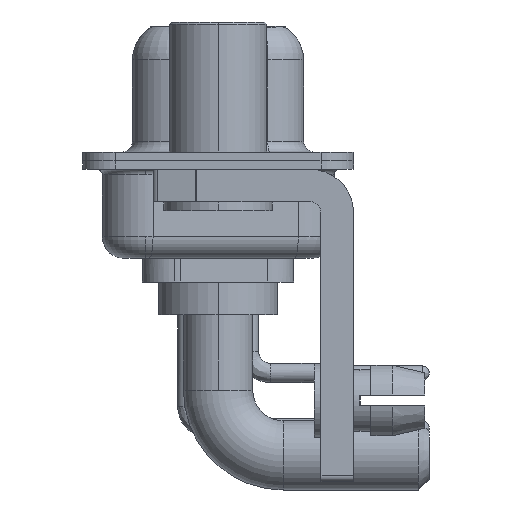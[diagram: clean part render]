
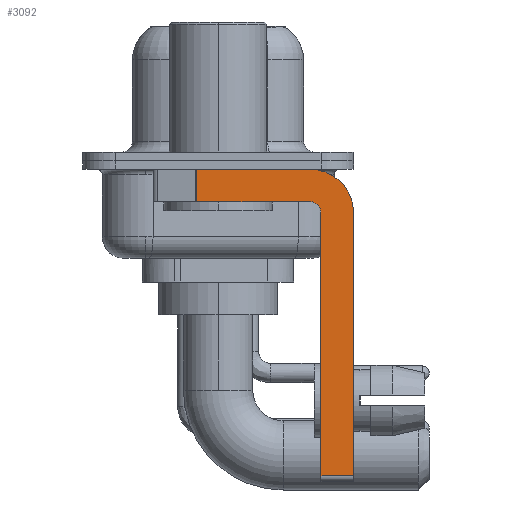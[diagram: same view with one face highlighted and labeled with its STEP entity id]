
A CAD part, left-side view. The second image highlights one B-rep face of the part: STEP entity #3092.
In plain terms, the highlighted planar face has unit normal (-1, 0, 0).
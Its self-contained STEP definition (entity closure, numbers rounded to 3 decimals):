
#45 = ORIENTED_EDGE ( 'NONE', *, *, #5757, .F. ) ;
#236 = LINE ( 'NONE', #1797, #17613 ) ;
#726 = CARTESIAN_POINT ( 'NONE',  ( -2.9, -4.25, -0.4 ) ) ;
#1777 = VERTEX_POINT ( 'NONE', #4942 ) ;
#1797 = CARTESIAN_POINT ( 'NONE',  ( -2.9, -4.25, -1.9 ) ) ;
#2208 = DIRECTION ( 'NONE',  ( 0., 0., -1. ) ) ;
#2331 = CIRCLE ( 'NONE', #6593, 2. ) ;
#2436 = EDGE_LOOP ( 'NONE', ( #10477, #22386, #17384, #18228, #45, #11481, #5623, #11283 ) ) ;
#3092 = ADVANCED_FACE ( 'NONE', ( #6260 ), #6143, .F. ) ;
#3889 = CARTESIAN_POINT ( 'NONE',  ( -2.9, -4.25, -14.55 ) ) ;
#4396 = VECTOR ( 'NONE', #17489, 1000. ) ;
#4942 = CARTESIAN_POINT ( 'NONE',  ( -2.9, -4.25, -1.9 ) ) ;
#5421 = DIRECTION ( 'NONE',  ( 0., 1., 0. ) ) ;
#5623 = ORIENTED_EDGE ( 'NONE', *, *, #12557, .F. ) ;
#5757 = EDGE_CURVE ( 'NONE', #8678, #9467, #18134, .T. ) ;
#5815 = CARTESIAN_POINT ( 'NONE',  ( -2.9, -6.25, -14.55 ) ) ;
#6081 = DIRECTION ( 'NONE',  ( 1., 0., 0. ) ) ;
#6143 = PLANE ( 'NONE',  #17071 ) ;
#6260 = FACE_OUTER_BOUND ( 'NONE', #2436, .T. ) ;
#6593 = AXIS2_PLACEMENT_3D ( 'NONE', #13405, #6081, #20726 ) ;
#6860 = DIRECTION ( 'NONE',  ( 0., 0., 1. ) ) ;
#6981 = CARTESIAN_POINT ( 'NONE',  ( -2.9, -4.75, -14.8 ) ) ;
#7157 = CARTESIAN_POINT ( 'NONE',  ( -2.9, -4.25, -2.4 ) ) ;
#7255 = VECTOR ( 'NONE', #2208, 1000. ) ;
#8071 = DIRECTION ( 'NONE',  ( 1., 0., 0. ) ) ;
#8337 = DIRECTION ( 'NONE',  ( 0., -1., 0. ) ) ;
#8678 = VERTEX_POINT ( 'NONE', #16023 ) ;
#8873 = EDGE_CURVE ( 'NONE', #9467, #1777, #18196, .T. ) ;
#9467 = VERTEX_POINT ( 'NONE', #22226 ) ;
#9577 = VECTOR ( 'NONE', #8337, 1000. ) ;
#10376 = CARTESIAN_POINT ( 'NONE',  ( -2.9, 3., -0.4 ) ) ;
#10477 = ORIENTED_EDGE ( 'NONE', *, *, #15186, .F. ) ;
#10492 = CARTESIAN_POINT ( 'NONE',  ( -2.9, 0.978, -0.4 ) ) ;
#11222 = VECTOR ( 'NONE', #6860, 1000. ) ;
#11283 = ORIENTED_EDGE ( 'NONE', *, *, #15885, .F. ) ;
#11481 = ORIENTED_EDGE ( 'NONE', *, *, #23567, .T. ) ;
#12557 = EDGE_CURVE ( 'NONE', #16480, #16474, #23639, .T. ) ;
#12675 = LINE ( 'NONE', #3889, #13358 ) ;
#12881 = DIRECTION ( 'NONE',  ( 0., 0., 1. ) ) ;
#13345 = DIRECTION ( 'NONE',  ( 0., 0., -1. ) ) ;
#13358 = VECTOR ( 'NONE', #20240, 1000. ) ;
#13375 = CARTESIAN_POINT ( 'NONE',  ( -2.9, -6.25, -2.4 ) ) ;
#13405 = CARTESIAN_POINT ( 'NONE',  ( -2.9, -4.25, -2.4 ) ) ;
#14865 = EDGE_CURVE ( 'NONE', #1777, #18834, #236, .T. ) ;
#15186 = EDGE_CURVE ( 'NONE', #16672, #15212, #19253, .T. ) ;
#15212 = VERTEX_POINT ( 'NONE', #726 ) ;
#15885 = EDGE_CURVE ( 'NONE', #15212, #16480, #2331, .T. ) ;
#16023 = CARTESIAN_POINT ( 'NONE',  ( -2.9, -4.75, -14.55 ) ) ;
#16474 = VERTEX_POINT ( 'NONE', #5815 ) ;
#16480 = VERTEX_POINT ( 'NONE', #13375 ) ;
#16672 = VERTEX_POINT ( 'NONE', #10492 ) ;
#17071 = AXIS2_PLACEMENT_3D ( 'NONE', #18644, #8071, #13345 ) ;
#17384 = ORIENTED_EDGE ( 'NONE', *, *, #14865, .F. ) ;
#17489 = DIRECTION ( 'NONE',  ( 0., 0., -1. ) ) ;
#17613 = VECTOR ( 'NONE', #5421, 1000. ) ;
#17819 = AXIS2_PLACEMENT_3D ( 'NONE', #7157, #20216, #12881 ) ;
#18134 = LINE ( 'NONE', #6981, #11222 ) ;
#18196 = CIRCLE ( 'NONE', #17819, 0.5 ) ;
#18228 = ORIENTED_EDGE ( 'NONE', *, *, #8873, .F. ) ;
#18644 = CARTESIAN_POINT ( 'NONE',  ( -2.9, -4.25, -2.4 ) ) ;
#18834 = VERTEX_POINT ( 'NONE', #21339 ) ;
#19144 = EDGE_CURVE ( 'NONE', #16672, #18834, #22879, .T. ) ;
#19253 = LINE ( 'NONE', #10376, #9577 ) ;
#19286 = CARTESIAN_POINT ( 'NONE',  ( -2.9, 0.978, -1.9 ) ) ;
#20216 = DIRECTION ( 'NONE',  ( -1., 0., 0. ) ) ;
#20240 = DIRECTION ( 'NONE',  ( 0., -1., 0. ) ) ;
#20726 = DIRECTION ( 'NONE',  ( 0., 0., -1. ) ) ;
#21339 = CARTESIAN_POINT ( 'NONE',  ( -2.9, 0.978, -1.9 ) ) ;
#22226 = CARTESIAN_POINT ( 'NONE',  ( -2.9, -4.75, -2.4 ) ) ;
#22386 = ORIENTED_EDGE ( 'NONE', *, *, #19144, .T. ) ;
#22879 = LINE ( 'NONE', #19286, #4396 ) ;
#23523 = CARTESIAN_POINT ( 'NONE',  ( -2.9, -6.25, -2.4 ) ) ;
#23567 = EDGE_CURVE ( 'NONE', #8678, #16474, #12675, .T. ) ;
#23639 = LINE ( 'NONE', #23523, #7255 ) ;
